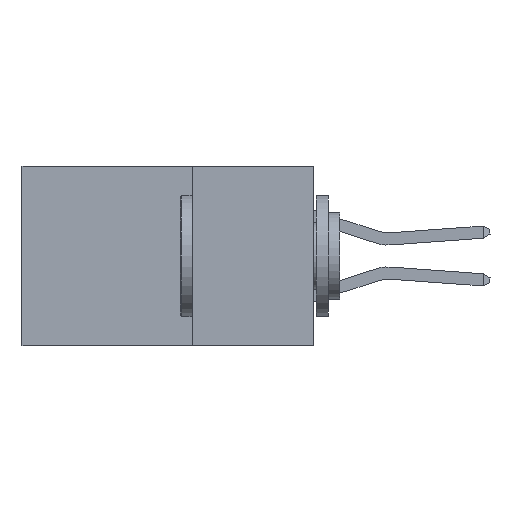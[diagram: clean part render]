
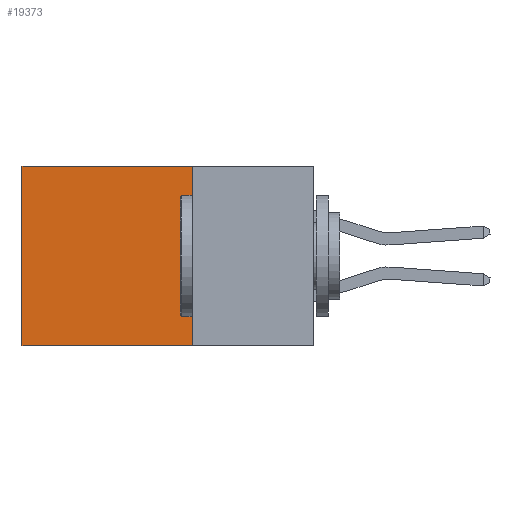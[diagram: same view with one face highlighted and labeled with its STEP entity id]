
A CAD part, left-side view. The second image highlights one B-rep face of the part: STEP entity #19373.
In plain terms, the highlighted planar face has unit normal (-1, 0, 0).
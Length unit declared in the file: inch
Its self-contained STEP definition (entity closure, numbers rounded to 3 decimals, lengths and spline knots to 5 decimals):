
#82 = DIRECTION ( 'NONE',  ( 0., 0., -1. ) ) ;
#802 = CARTESIAN_POINT ( 'NONE',  ( 0.2875, 0.6, 0. ) ) ;
#834 = VERTEX_POINT ( 'NONE', #802 ) ;
#1678 = FACE_OUTER_BOUND ( 'NONE', #26696, .T. ) ;
#2453 = DIRECTION ( 'NONE',  ( 0., 0., -1. ) ) ;
#2995 = VERTEX_POINT ( 'NONE', #26753 ) ;
#3204 = DIRECTION ( 'NONE',  ( 0., 1., 0. ) ) ;
#3567 = CARTESIAN_POINT ( 'NONE',  ( 0.2875, 0.25, 0. ) ) ;
#4196 = EDGE_CURVE ( 'NONE', #834, #5847, #18611, .T. ) ;
#4220 = LINE ( 'NONE', #22092, #22275 ) ;
#4238 = ORIENTED_EDGE ( 'NONE', *, *, #16481, .F. ) ;
#5847 = VERTEX_POINT ( 'NONE', #18035 ) ;
#6097 = VECTOR ( 'NONE', #82, 39.37008 ) ;
#8904 = CARTESIAN_POINT ( 'NONE',  ( 0.2875, 0.25, 0. ) ) ;
#9073 = CARTESIAN_POINT ( 'NONE',  ( 0.2875, 0.25, 0. ) ) ;
#10709 = LINE ( 'NONE', #3567, #17645 ) ;
#12453 = VERTEX_POINT ( 'NONE', #9073 ) ;
#14371 = CARTESIAN_POINT ( 'NONE',  ( 0.2875, 0.25, 0. ) ) ;
#16054 = EDGE_CURVE ( 'NONE', #12453, #834, #28425, .T. ) ;
#16481 = EDGE_CURVE ( 'NONE', #12453, #2995, #10709, .T. ) ;
#16709 = PLANE ( 'NONE',  #27686 ) ;
#16803 = DIRECTION ( 'NONE',  ( 1., 0., 0. ) ) ;
#17571 = EDGE_CURVE ( 'NONE', #2995, #5847, #4220, .T. ) ;
#17645 = VECTOR ( 'NONE', #20159, 39.37008 ) ;
#18035 = CARTESIAN_POINT ( 'NONE',  ( 0.2875, 0.6, -0.37 ) ) ;
#18611 = LINE ( 'NONE', #19242, #6097 ) ;
#19242 = CARTESIAN_POINT ( 'NONE',  ( 0.2875, 0.6, 0. ) ) ;
#19373 = ADVANCED_FACE ( 'NONE', ( #1678 ), #16709, .F. ) ;
#20159 = DIRECTION ( 'NONE',  ( 0., 0., -1. ) ) ;
#22092 = CARTESIAN_POINT ( 'NONE',  ( 0.2875, 0.25, -0.37 ) ) ;
#22275 = VECTOR ( 'NONE', #3204, 39.37008 ) ;
#22635 = ORIENTED_EDGE ( 'NONE', *, *, #4196, .T. ) ;
#23848 = ORIENTED_EDGE ( 'NONE', *, *, #16054, .T. ) ;
#24651 = ORIENTED_EDGE ( 'NONE', *, *, #17571, .F. ) ;
#26696 = EDGE_LOOP ( 'NONE', ( #22635, #24651, #4238, #23848 ) ) ;
#26753 = CARTESIAN_POINT ( 'NONE',  ( 0.2875, 0.25, -0.37 ) ) ;
#27420 = DIRECTION ( 'NONE',  ( 0., 1., 0. ) ) ;
#27686 = AXIS2_PLACEMENT_3D ( 'NONE', #14371, #16803, #2453 ) ;
#27691 = VECTOR ( 'NONE', #27420, 39.37008 ) ;
#28425 = LINE ( 'NONE', #8904, #27691 ) ;
